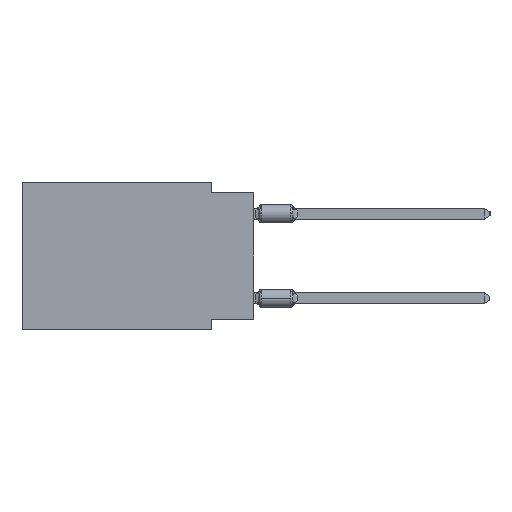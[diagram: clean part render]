
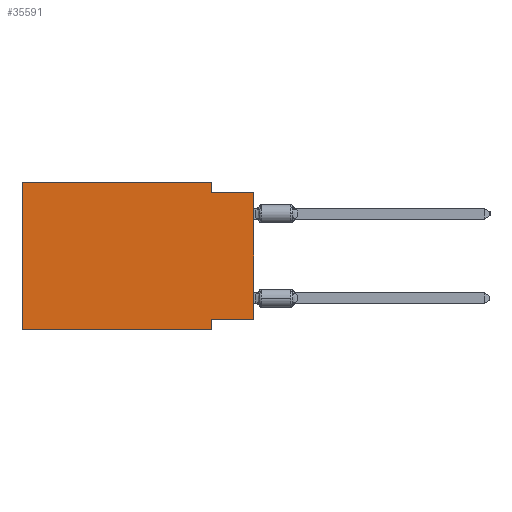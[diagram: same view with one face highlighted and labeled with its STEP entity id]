
A CAD part, left-side view. The second image highlights one B-rep face of the part: STEP entity #35591.
In plain terms, the highlighted planar face has unit normal (-1, 0, 0).
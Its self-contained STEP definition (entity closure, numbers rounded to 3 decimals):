
#457 = LINE ( 'NONE', #5612, #43598 ) ;
#794 = CARTESIAN_POINT ( 'NONE',  ( 0., 13.97, 0. ) ) ;
#973 = ORIENTED_EDGE ( 'NONE', *, *, #46753, .F. ) ;
#2062 = CARTESIAN_POINT ( 'NONE',  ( 0., 2.54, -8.255 ) ) ;
#2359 = VECTOR ( 'NONE', #3305, 1000. ) ;
#2456 = EDGE_LOOP ( 'NONE', ( #54833, #38685, #31573, #25778, #51617, #7241, #6763, #973 ) ) ;
#3305 = DIRECTION ( 'NONE',  ( 0., -1., 0. ) ) ;
#5612 = CARTESIAN_POINT ( 'NONE',  ( 0., 2.54, 0. ) ) ;
#5890 = EDGE_CURVE ( 'NONE', #11332, #52423, #21517, .T. ) ;
#6763 = ORIENTED_EDGE ( 'NONE', *, *, #43730, .F. ) ;
#6868 = EDGE_CURVE ( 'NONE', #52423, #57107, #457, .T. ) ;
#7241 = ORIENTED_EDGE ( 'NONE', *, *, #38212, .T. ) ;
#7680 = CARTESIAN_POINT ( 'NONE',  ( 0., 2.54, -0.635 ) ) ;
#10567 = DIRECTION ( 'NONE',  ( 0., -1., 0. ) ) ;
#11332 = VERTEX_POINT ( 'NONE', #794 ) ;
#12674 = CARTESIAN_POINT ( 'NONE',  ( 0., 0., -0.635 ) ) ;
#12701 = FACE_OUTER_BOUND ( 'NONE', #2456, .T. ) ;
#13617 = CARTESIAN_POINT ( 'NONE',  ( 0., 0., -8.255 ) ) ;
#14363 = CARTESIAN_POINT ( 'NONE',  ( 0., 0., -0.635 ) ) ;
#15301 = DIRECTION ( 'NONE',  ( 0., 0., -1. ) ) ;
#15302 = DIRECTION ( 'NONE',  ( 0., 0., 1. ) ) ;
#16457 = VECTOR ( 'NONE', #16997, 1000. ) ;
#16997 = DIRECTION ( 'NONE',  ( 0., -1., 0. ) ) ;
#17837 = CARTESIAN_POINT ( 'NONE',  ( 0., 13.97, 0. ) ) ;
#18694 = VECTOR ( 'NONE', #27248, 1000. ) ;
#19098 = LINE ( 'NONE', #13617, #18694 ) ;
#21257 = CARTESIAN_POINT ( 'NONE',  ( 0., 2.54, 0. ) ) ;
#21517 = LINE ( 'NONE', #58463, #16457 ) ;
#22084 = DIRECTION ( 'NONE',  ( 0., 0., -1. ) ) ;
#24160 = LINE ( 'NONE', #28419, #58755 ) ;
#24669 = CARTESIAN_POINT ( 'NONE',  ( 0., 13.97, 0. ) ) ;
#25778 = ORIENTED_EDGE ( 'NONE', *, *, #5890, .F. ) ;
#26287 = CARTESIAN_POINT ( 'NONE',  ( 0., 13.97, -8.89 ) ) ;
#27248 = DIRECTION ( 'NONE',  ( 0., 1., 0. ) ) ;
#28419 = CARTESIAN_POINT ( 'NONE',  ( 0., 13.97, -8.89 ) ) ;
#30025 = VERTEX_POINT ( 'NONE', #26287 ) ;
#31160 = PLANE ( 'NONE',  #49844 ) ;
#31389 = VECTOR ( 'NONE', #44101, 1000. ) ;
#31573 = ORIENTED_EDGE ( 'NONE', *, *, #6868, .F. ) ;
#34647 = VERTEX_POINT ( 'NONE', #2062 ) ;
#34658 = LINE ( 'NONE', #24669, #39912 ) ;
#35591 = ADVANCED_FACE ( 'NONE', ( #12701 ), #31160, .F. ) ;
#35798 = CARTESIAN_POINT ( 'NONE',  ( 0., 2.54, -8.89 ) ) ;
#35975 = LINE ( 'NONE', #12674, #2359 ) ;
#38212 = EDGE_CURVE ( 'NONE', #30025, #46140, #24160, .T. ) ;
#38685 = ORIENTED_EDGE ( 'NONE', *, *, #59049, .F. ) ;
#39746 = LINE ( 'NONE', #35798, #58355 ) ;
#39912 = VECTOR ( 'NONE', #15302, 1000. ) ;
#41468 = VERTEX_POINT ( 'NONE', #47872 ) ;
#43508 = LINE ( 'NONE', #53774, #31389 ) ;
#43598 = VECTOR ( 'NONE', #15301, 1000. ) ;
#43730 = EDGE_CURVE ( 'NONE', #34647, #46140, #39746, .T. ) ;
#44101 = DIRECTION ( 'NONE',  ( 0., 0., 1. ) ) ;
#46140 = VERTEX_POINT ( 'NONE', #51927 ) ;
#46149 = EDGE_CURVE ( 'NONE', #30025, #11332, #34658, .T. ) ;
#46753 = EDGE_CURVE ( 'NONE', #41468, #34647, #19098, .T. ) ;
#47872 = CARTESIAN_POINT ( 'NONE',  ( 0., 0., -8.255 ) ) ;
#49636 = DIRECTION ( 'NONE',  ( 1., 0., 0. ) ) ;
#49844 = AXIS2_PLACEMENT_3D ( 'NONE', #17837, #49636, #22084 ) ;
#51617 = ORIENTED_EDGE ( 'NONE', *, *, #46149, .F. ) ;
#51927 = CARTESIAN_POINT ( 'NONE',  ( 0., 2.54, -8.89 ) ) ;
#52214 = VERTEX_POINT ( 'NONE', #14363 ) ;
#52423 = VERTEX_POINT ( 'NONE', #21257 ) ;
#53774 = CARTESIAN_POINT ( 'NONE',  ( 0., 0., 0. ) ) ;
#54833 = ORIENTED_EDGE ( 'NONE', *, *, #58237, .T. ) ;
#57107 = VERTEX_POINT ( 'NONE', #7680 ) ;
#58237 = EDGE_CURVE ( 'NONE', #41468, #52214, #43508, .T. ) ;
#58355 = VECTOR ( 'NONE', #58521, 1000. ) ;
#58463 = CARTESIAN_POINT ( 'NONE',  ( 0., 13.97, 0. ) ) ;
#58521 = DIRECTION ( 'NONE',  ( 0., 0., -1. ) ) ;
#58755 = VECTOR ( 'NONE', #10567, 1000. ) ;
#59049 = EDGE_CURVE ( 'NONE', #57107, #52214, #35975, .T. ) ;
